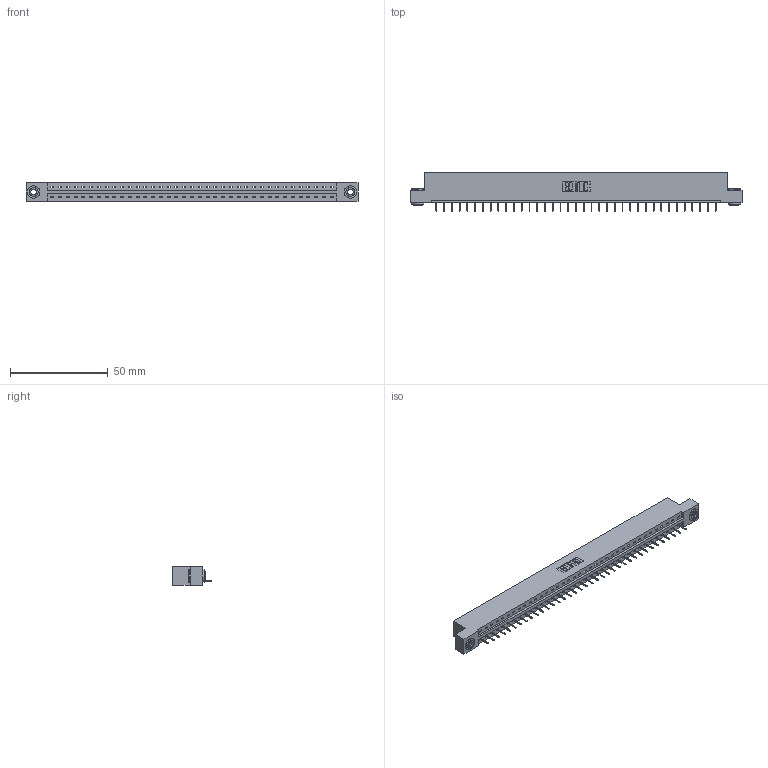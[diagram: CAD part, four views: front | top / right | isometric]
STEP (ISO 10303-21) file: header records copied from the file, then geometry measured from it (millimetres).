
FILE_DESCRIPTION (( 'STEP AP203' ), '1' );
FILE_NAME ('337-037-524-103.STEP', '2019-10-01T15:23:41', ( '' ), ( '' ), 'SwSTEP 2.0', 'SolidWorks 2016', '' );
FILE_SCHEMA (( 'CONFIG_CONTROL_DESIGN' ));
Length unit declared in the file: inch
Products named in the file (4): 345-292-001_345-293-124; 337 Part_Flush Mounting Lugs - 0.156 Dia-TH; 345-250-002_345-250-002-102; 337-037-524-103
Assembly tree (40 placements, depth 2):
  337-037-524-103
    337 Part_Flush Mounting Lugs - 0.156 Dia-TH
    345-292-001_345-293-124  x37
    345-250-002_345-250-002-102  x2
Bounding box: 169.62 x 19.69 x 9.4 mm (x, y, z)
Volume: 17439.9 mm3; surface area: 17712.6 mm2
Topology: 40 solids, 40 shells, 2594 faces, 7491 edges, 4842 vertices
Faces by surface type: plane 2004, cylinder 582, cone 8
Entity records: 28874 total; most frequent: CARTESIAN_POINT 5004, ORIENTED_EDGE 4970, DIRECTION 4257, EDGE_CURVE 2485, LINE 2337, VECTOR 2337, VERTEX_POINT 1650, AXIS2_PLACEMENT_3D 960
